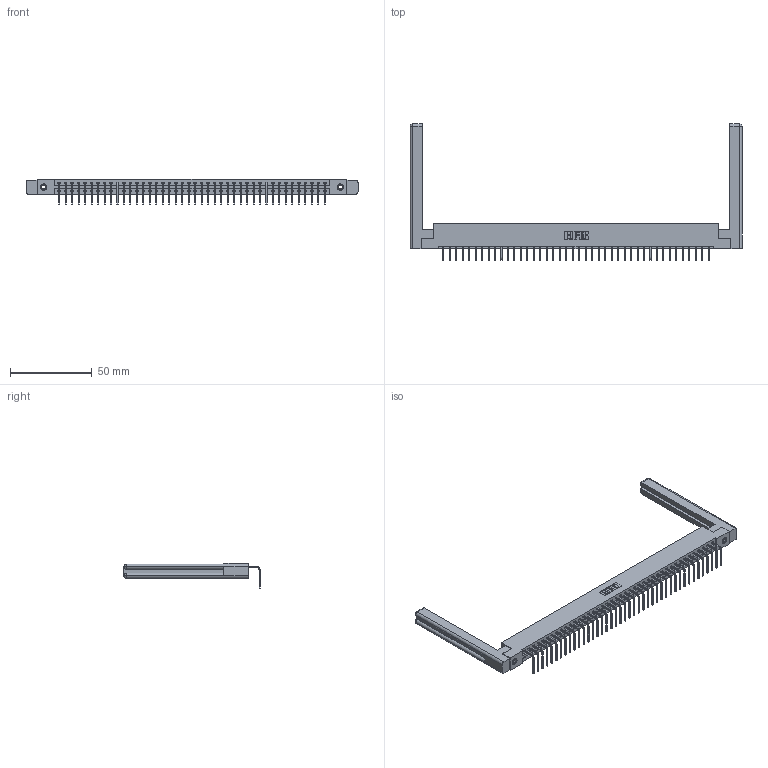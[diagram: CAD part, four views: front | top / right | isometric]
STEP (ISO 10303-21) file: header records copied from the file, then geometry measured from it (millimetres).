
FILE_DESCRIPTION (( 'STEP AP203' ), '1' );
FILE_NAME ('387-042-558-158.STEP', '2019-10-07T21:50:30', ( '' ), ( '' ), 'SwSTEP 2.0', 'SolidWorks 2016', '' );
FILE_SCHEMA (( 'CONFIG_CONTROL_DESIGN' ));
Length unit declared in the file: inch
Products named in the file (5): 345-292-001_558 Tail - 2; 345-250-001_345-250-001-102; 387-042-558-158; 307-220-058; 337 Part_Flush Mounting Lugs - 0.156 Dia-TI
Assembly tree (47 placements, depth 2):
  387-042-558-158
    337 Part_Flush Mounting Lugs - 0.156 Dia-TI
    345-292-001_558 Tail - 2  x42
    345-250-001_345-250-001-102  x2
    307-220-058  x2
Bounding box: 203.05 x 83.25 x 15.37 mm (x, y, z)
Volume: 28405.5 mm3; surface area: 28024.6 mm2
Topology: 47 solids, 47 shells, 2944 faces, 8813 edges, 5806 vertices
Faces by surface type: plane 2170, cylinder 750, cone 12, torus 12
Entity records: 33938 total; most frequent: CARTESIAN_POINT 5911, ORIENTED_EDGE 5828, DIRECTION 4994, EDGE_CURVE 2914, VECTOR 2738, LINE 2738, VERTEX_POINT 1934, AXIS2_PLACEMENT_3D 1128
